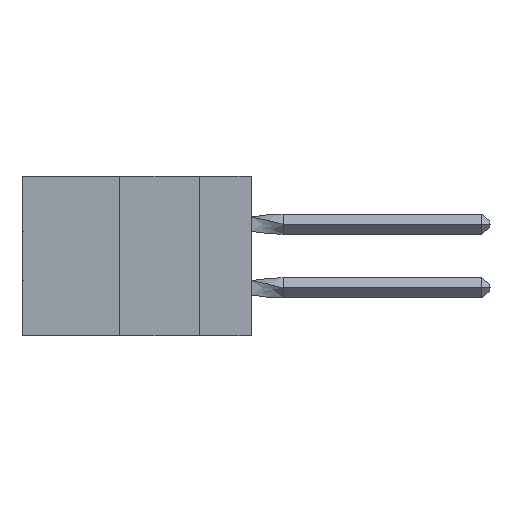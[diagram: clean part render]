
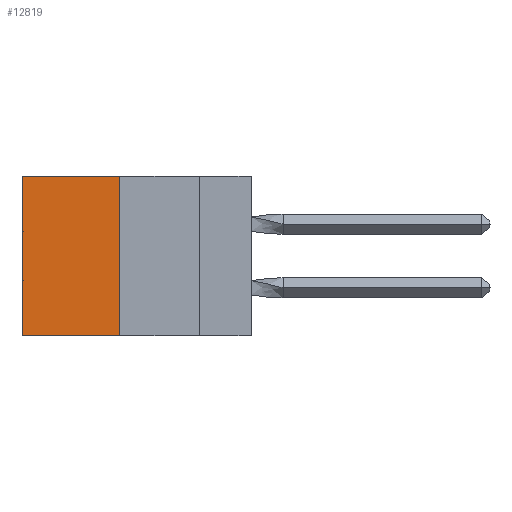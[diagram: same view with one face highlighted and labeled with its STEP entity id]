
A CAD part, left-side view. The second image highlights one B-rep face of the part: STEP entity #12819.
In plain terms, the highlighted planar face has unit normal (-1, 0, 0).
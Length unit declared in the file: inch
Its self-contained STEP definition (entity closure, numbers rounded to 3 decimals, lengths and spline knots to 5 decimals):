
#487 = CARTESIAN_POINT ( 'NONE',  ( 0.305, 0.72, -0.5 ) ) ;
#585 = VECTOR ( 'NONE', #6233, 39.37008 ) ;
#974 = LINE ( 'NONE', #3969, #32233 ) ;
#1812 = DIRECTION ( 'NONE',  ( 0., 0., -1. ) ) ;
#3969 = CARTESIAN_POINT ( 'NONE',  ( 0.305, 0.413, 0. ) ) ;
#4008 = CARTESIAN_POINT ( 'NONE',  ( 0.305, 0.72, 0. ) ) ;
#6170 = ORIENTED_EDGE ( 'NONE', *, *, #14200, .F. ) ;
#6233 = DIRECTION ( 'NONE',  ( 0., 1., 0. ) ) ;
#7704 = DIRECTION ( 'NONE',  ( 0., 0., -1. ) ) ;
#9952 = VECTOR ( 'NONE', #7704, 39.37008 ) ;
#9978 = EDGE_LOOP ( 'NONE', ( #17849, #39329, #6170, #22290 ) ) ;
#10881 = LINE ( 'NONE', #33648, #25910 ) ;
#11082 = EDGE_CURVE ( 'NONE', #13988, #31073, #18307, .T. ) ;
#11546 = VERTEX_POINT ( 'NONE', #39160 ) ;
#12819 = ADVANCED_FACE ( 'NONE', ( #27382 ), #32409, .F. ) ;
#13988 = VERTEX_POINT ( 'NONE', #4008 ) ;
#14200 = EDGE_CURVE ( 'NONE', #33213, #11546, #10881, .T. ) ;
#14776 = DIRECTION ( 'NONE',  ( 0., 1., 0. ) ) ;
#17849 = ORIENTED_EDGE ( 'NONE', *, *, #11082, .T. ) ;
#18307 = LINE ( 'NONE', #487, #9952 ) ;
#20787 = CARTESIAN_POINT ( 'NONE',  ( 0.305, 0.72, -0.5 ) ) ;
#22290 = ORIENTED_EDGE ( 'NONE', *, *, #31216, .T. ) ;
#22464 = CARTESIAN_POINT ( 'NONE',  ( 0.305, 0.413, -0.5 ) ) ;
#24495 = CARTESIAN_POINT ( 'NONE',  ( 0.305, 0.413, 0. ) ) ;
#25910 = VECTOR ( 'NONE', #1812, 39.37008 ) ;
#27382 = FACE_OUTER_BOUND ( 'NONE', #9978, .T. ) ;
#31073 = VERTEX_POINT ( 'NONE', #20787 ) ;
#31216 = EDGE_CURVE ( 'NONE', #33213, #13988, #974, .T. ) ;
#31306 = LINE ( 'NONE', #34324, #585 ) ;
#32233 = VECTOR ( 'NONE', #14776, 39.37008 ) ;
#32409 = PLANE ( 'NONE',  #41257 ) ;
#32875 = DIRECTION ( 'NONE',  ( 1., 0., 0. ) ) ;
#33213 = VERTEX_POINT ( 'NONE', #24495 ) ;
#33648 = CARTESIAN_POINT ( 'NONE',  ( 0.305, 0.413, -0.5 ) ) ;
#34324 = CARTESIAN_POINT ( 'NONE',  ( 0.305, 0.413, -0.5 ) ) ;
#38927 = EDGE_CURVE ( 'NONE', #11546, #31073, #31306, .T. ) ;
#39160 = CARTESIAN_POINT ( 'NONE',  ( 0.305, 0.413, -0.5 ) ) ;
#39329 = ORIENTED_EDGE ( 'NONE', *, *, #38927, .F. ) ;
#40056 = DIRECTION ( 'NONE',  ( 0., 0., -1. ) ) ;
#41257 = AXIS2_PLACEMENT_3D ( 'NONE', #22464, #32875, #40056 ) ;
